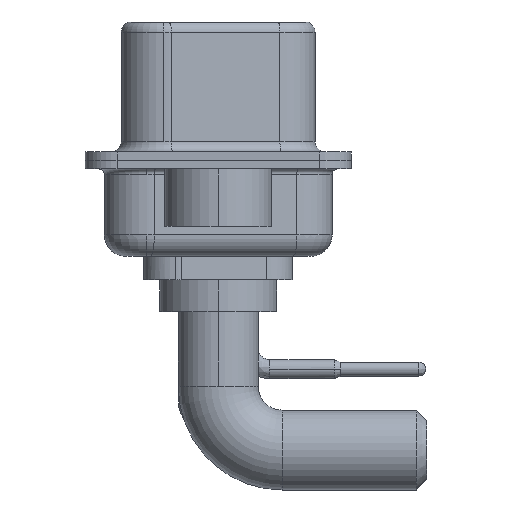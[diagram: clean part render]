
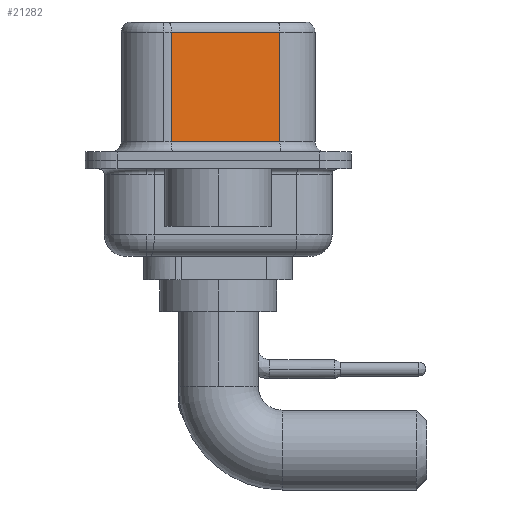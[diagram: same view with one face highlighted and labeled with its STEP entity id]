
A CAD part, left-side view. The second image highlights one B-rep face of the part: STEP entity #21282.
In plain terms, the highlighted planar face has unit normal (-0.985, -0.174, 0).
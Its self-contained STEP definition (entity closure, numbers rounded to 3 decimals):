
#130 = VERTEX_POINT ( 'NONE', #20897 ) ;
#425 = VECTOR ( 'NONE', #8652, 1000. ) ;
#488 = LINE ( 'NONE', #13518, #13812 ) ;
#841 = DIRECTION ( 'NONE',  ( -0.174, 0.985, 0. ) ) ;
#1073 = EDGE_CURVE ( 'NONE', #20255, #130, #13988, .T. ) ;
#1217 = EDGE_LOOP ( 'NONE', ( #17455, #23238, #11085, #20183 ) ) ;
#1251 = DIRECTION ( 'NONE',  ( 0.985, 0.174, 0. ) ) ;
#2711 = DIRECTION ( 'NONE',  ( -0.174, 0.985, 0. ) ) ;
#2858 = VECTOR ( 'NONE', #841, 1000. ) ;
#3265 = LINE ( 'NONE', #14241, #18753 ) ;
#4321 = EDGE_CURVE ( 'NONE', #6974, #12574, #488, .T. ) ;
#4950 = CARTESIAN_POINT ( 'NONE',  ( 3.68, 2.203, 6.52 ) ) ;
#6626 = FACE_OUTER_BOUND ( 'NONE', #1217, .T. ) ;
#6974 = VERTEX_POINT ( 'NONE', #11678 ) ;
#8652 = DIRECTION ( 'NONE',  ( 0., 0., -1. ) ) ;
#9814 = DIRECTION ( 'NONE',  ( 0.174, -0.985, 0. ) ) ;
#11085 = ORIENTED_EDGE ( 'NONE', *, *, #23449, .T. ) ;
#11678 = CARTESIAN_POINT ( 'NONE',  ( 3.68, 2.203, 0.9 ) ) ;
#12001 = CARTESIAN_POINT ( 'NONE',  ( 4.58, -2.897, 6.52 ) ) ;
#12459 = DIRECTION ( 'NONE',  ( 0., 0., -1. ) ) ;
#12574 = VERTEX_POINT ( 'NONE', #19128 ) ;
#13518 = CARTESIAN_POINT ( 'NONE',  ( 4.58, -2.897, 0.9 ) ) ;
#13812 = VECTOR ( 'NONE', #9814, 1000. ) ;
#13988 = LINE ( 'NONE', #15657, #2858 ) ;
#14241 = CARTESIAN_POINT ( 'NONE',  ( 4.58, -2.897, 6.52 ) ) ;
#15657 = CARTESIAN_POINT ( 'NONE',  ( 4.58, -2.897, 6.02 ) ) ;
#15672 = AXIS2_PLACEMENT_3D ( 'NONE', #12001, #1251, #2711 ) ;
#17455 = ORIENTED_EDGE ( 'NONE', *, *, #22031, .F. ) ;
#17518 = PLANE ( 'NONE',  #15672 ) ;
#17849 = LINE ( 'NONE', #4950, #425 ) ;
#18753 = VECTOR ( 'NONE', #12459, 1000. ) ;
#19128 = CARTESIAN_POINT ( 'NONE',  ( 4.58, -2.897, 0.9 ) ) ;
#19334 = CARTESIAN_POINT ( 'NONE',  ( 4.58, -2.897, 6.02 ) ) ;
#20183 = ORIENTED_EDGE ( 'NONE', *, *, #4321, .T. ) ;
#20255 = VERTEX_POINT ( 'NONE', #19334 ) ;
#20897 = CARTESIAN_POINT ( 'NONE',  ( 3.68, 2.203, 6.02 ) ) ;
#21282 = ADVANCED_FACE ( 'NONE', ( #6626 ), #17518, .F. ) ;
#22031 = EDGE_CURVE ( 'NONE', #20255, #12574, #3265, .T. ) ;
#23238 = ORIENTED_EDGE ( 'NONE', *, *, #1073, .T. ) ;
#23449 = EDGE_CURVE ( 'NONE', #130, #6974, #17849, .T. ) ;
